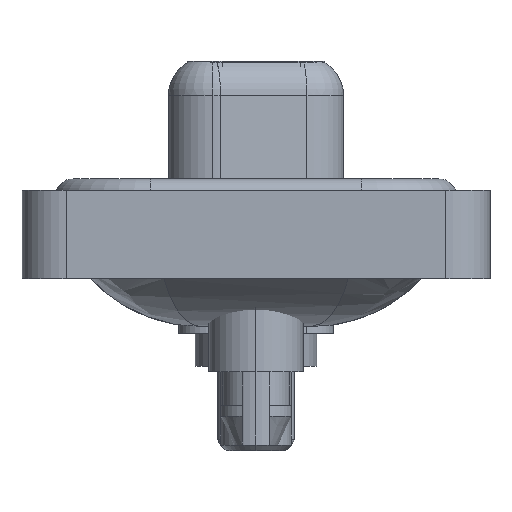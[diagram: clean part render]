
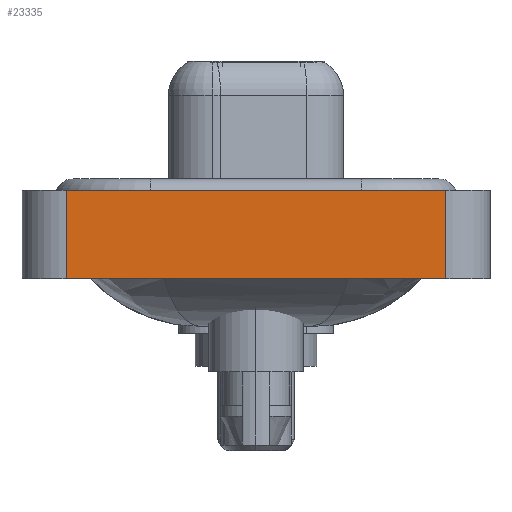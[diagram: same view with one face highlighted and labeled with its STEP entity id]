
A CAD part, left-side view. The second image highlights one B-rep face of the part: STEP entity #23335.
In plain terms, the highlighted planar face has unit normal (-1, 0, 0).
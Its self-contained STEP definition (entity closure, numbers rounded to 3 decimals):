
#1644 = ORIENTED_EDGE ( 'NONE', *, *, #7985, .T. ) ;
#2161 = EDGE_LOOP ( 'NONE', ( #1644, #3579, #23257, #11105 ) ) ;
#2231 = CARTESIAN_POINT ( 'NONE',  ( -7.35, -8.55, -3.6 ) ) ;
#2555 = VERTEX_POINT ( 'NONE', #14426 ) ;
#3507 = LINE ( 'NONE', #14396, #4764 ) ;
#3579 = ORIENTED_EDGE ( 'NONE', *, *, #21990, .F. ) ;
#3584 = DIRECTION ( 'NONE',  ( 0., 0., 1. ) ) ;
#4258 = EDGE_CURVE ( 'NONE', #14988, #2555, #3507, .T. ) ;
#4423 = CARTESIAN_POINT ( 'NONE',  ( -7.35, 8.55, 0.4 ) ) ;
#4764 = VECTOR ( 'NONE', #8817, 1000. ) ;
#5669 = AXIS2_PLACEMENT_3D ( 'NONE', #8185, #17286, #3584 ) ;
#5786 = DIRECTION ( 'NONE',  ( 0., 0., 1. ) ) ;
#5906 = DIRECTION ( 'NONE',  ( 0., 0., 1. ) ) ;
#7253 = CARTESIAN_POINT ( 'NONE',  ( -7.35, -8.55, 0.4 ) ) ;
#7985 = EDGE_CURVE ( 'NONE', #2555, #12480, #8972, .T. ) ;
#8185 = CARTESIAN_POINT ( 'NONE',  ( -7.35, -8.55, -3.6 ) ) ;
#8745 = LINE ( 'NONE', #21172, #20134 ) ;
#8817 = DIRECTION ( 'NONE',  ( 0., -1., 0. ) ) ;
#8972 = LINE ( 'NONE', #2231, #20332 ) ;
#9948 = PLANE ( 'NONE',  #5669 ) ;
#10632 = LINE ( 'NONE', #10981, #14331 ) ;
#10981 = CARTESIAN_POINT ( 'NONE',  ( -7.35, 8.55, -3.6 ) ) ;
#11105 = ORIENTED_EDGE ( 'NONE', *, *, #4258, .T. ) ;
#12480 = VERTEX_POINT ( 'NONE', #7253 ) ;
#14331 = VECTOR ( 'NONE', #5786, 1000. ) ;
#14396 = CARTESIAN_POINT ( 'NONE',  ( -7.35, -8.55, -3.6 ) ) ;
#14426 = CARTESIAN_POINT ( 'NONE',  ( -7.35, -8.55, -3.6 ) ) ;
#14988 = VERTEX_POINT ( 'NONE', #17738 ) ;
#17286 = DIRECTION ( 'NONE',  ( -1., 0., 0. ) ) ;
#17738 = CARTESIAN_POINT ( 'NONE',  ( -7.35, 8.55, -3.6 ) ) ;
#17845 = DIRECTION ( 'NONE',  ( 0., -1., 0. ) ) ;
#19265 = EDGE_CURVE ( 'NONE', #14988, #23110, #10632, .T. ) ;
#20134 = VECTOR ( 'NONE', #17845, 1000. ) ;
#20332 = VECTOR ( 'NONE', #5906, 1000. ) ;
#21172 = CARTESIAN_POINT ( 'NONE',  ( -7.35, -8.55, 0.4 ) ) ;
#21990 = EDGE_CURVE ( 'NONE', #23110, #12480, #8745, .T. ) ;
#22992 = FACE_OUTER_BOUND ( 'NONE', #2161, .T. ) ;
#23110 = VERTEX_POINT ( 'NONE', #4423 ) ;
#23257 = ORIENTED_EDGE ( 'NONE', *, *, #19265, .F. ) ;
#23335 = ADVANCED_FACE ( 'NONE', ( #22992 ), #9948, .T. ) ;
